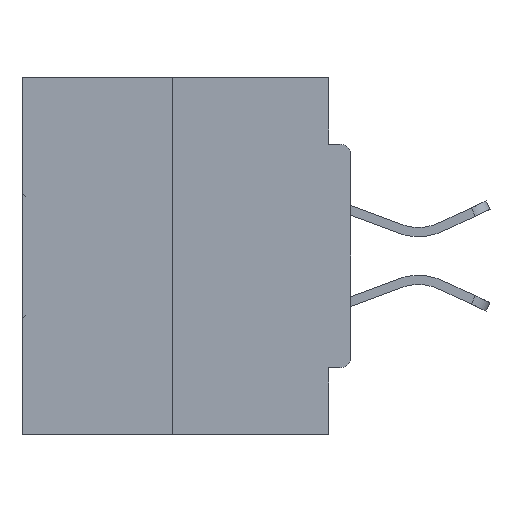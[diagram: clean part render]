
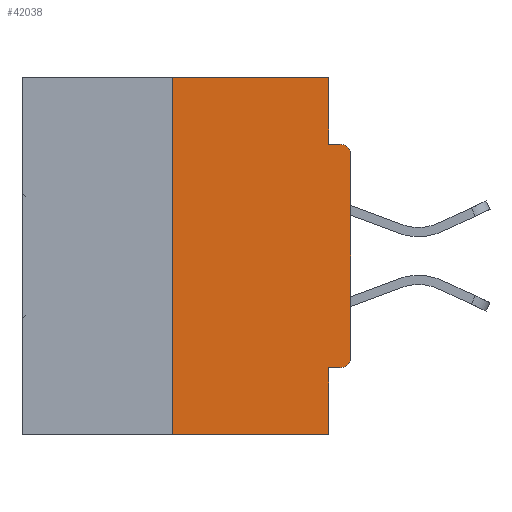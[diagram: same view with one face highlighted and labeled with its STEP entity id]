
A CAD part, left-side view. The second image highlights one B-rep face of the part: STEP entity #42038.
In plain terms, the highlighted planar face has unit normal (-1, 0, 0).
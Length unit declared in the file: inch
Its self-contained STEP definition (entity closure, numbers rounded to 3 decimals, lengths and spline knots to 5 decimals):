
#334 = DIRECTION ( 'NONE',  ( 0., 0., -1. ) ) ;
#1016 = VERTEX_POINT ( 'NONE', #9469 ) ;
#1318 = DIRECTION ( 'NONE',  ( 0., 1., 0. ) ) ;
#1459 = DIRECTION ( 'NONE',  ( 0., 0., -1. ) ) ;
#1527 = AXIS2_PLACEMENT_3D ( 'NONE', #21314, #37985, #27850 ) ;
#2402 = VERTEX_POINT ( 'NONE', #4307 ) ;
#3117 = CARTESIAN_POINT ( 'NONE',  ( 0., 0.031, 0. ) ) ;
#3133 = ORIENTED_EDGE ( 'NONE', *, *, #43009, .T. ) ;
#3311 = VECTOR ( 'NONE', #43446, 39.37008 ) ;
#3558 = ORIENTED_EDGE ( 'NONE', *, *, #34894, .F. ) ;
#3922 = PLANE ( 'NONE',  #1527 ) ;
#4307 = CARTESIAN_POINT ( 'NONE',  ( 0., 0.25, -0.5 ) ) ;
#4347 = EDGE_CURVE ( 'NONE', #12776, #28680, #35687, .T. ) ;
#4463 = ORIENTED_EDGE ( 'NONE', *, *, #4347, .T. ) ;
#5282 = EDGE_CURVE ( 'NONE', #12776, #1016, #42482, .T. ) ;
#5519 = CARTESIAN_POINT ( 'NONE',  ( 0., 0.015, -0.0935 ) ) ;
#5684 = VERTEX_POINT ( 'NONE', #11713 ) ;
#5718 = VECTOR ( 'NONE', #26559, 39.37008 ) ;
#6211 = CARTESIAN_POINT ( 'NONE',  ( 0., 0.25, 0. ) ) ;
#6405 = VECTOR ( 'NONE', #334, 39.37008 ) ;
#7506 = ORIENTED_EDGE ( 'NONE', *, *, #43290, .T. ) ;
#7690 = VERTEX_POINT ( 'NONE', #5519 ) ;
#8059 = LINE ( 'NONE', #3117, #6405 ) ;
#9285 = CARTESIAN_POINT ( 'NONE',  ( 0., 0.031, -0.5 ) ) ;
#9469 = CARTESIAN_POINT ( 'NONE',  ( 0., 0.031, -0.4065 ) ) ;
#10117 = LINE ( 'NONE', #15519, #36185 ) ;
#10723 = CARTESIAN_POINT ( 'NONE',  ( 0., 0.031, -0.5 ) ) ;
#11568 = CARTESIAN_POINT ( 'NONE',  ( 0., 0.015, -0.4065 ) ) ;
#11713 = CARTESIAN_POINT ( 'NONE',  ( 0., 0., -0.1085 ) ) ;
#12007 = CARTESIAN_POINT ( 'NONE',  ( 0., 0.031, 0. ) ) ;
#12776 = VERTEX_POINT ( 'NONE', #11568 ) ;
#13232 = EDGE_LOOP ( 'NONE', ( #34728, #21912, #25140, #3558, #31041, #4463, #7506, #3133, #35526, #29501 ) ) ;
#13595 = DIRECTION ( 'NONE',  ( -1., 0., 0. ) ) ;
#14269 = DIRECTION ( 'NONE',  ( 0., 0., -1. ) ) ;
#14966 = VERTEX_POINT ( 'NONE', #22808 ) ;
#15519 = CARTESIAN_POINT ( 'NONE',  ( 0., 0., -0.0935 ) ) ;
#16822 = CARTESIAN_POINT ( 'NONE',  ( 0., 0.46, -0.5 ) ) ;
#17137 = CIRCLE ( 'NONE', #24014, 0.015 ) ;
#18569 = DIRECTION ( 'NONE',  ( 0., -1., 0. ) ) ;
#20213 = VECTOR ( 'NONE', #43992, 39.37008 ) ;
#20291 = AXIS2_PLACEMENT_3D ( 'NONE', #22731, #13595, #14269 ) ;
#20331 = EDGE_CURVE ( 'NONE', #37708, #37813, #36535, .T. ) ;
#21314 = CARTESIAN_POINT ( 'NONE',  ( 0., 0.46, 0. ) ) ;
#21371 = DIRECTION ( 'NONE',  ( -1., 0., 0. ) ) ;
#21415 = LINE ( 'NONE', #36383, #3311 ) ;
#21912 = ORIENTED_EDGE ( 'NONE', *, *, #25961, .F. ) ;
#22731 = CARTESIAN_POINT ( 'NONE',  ( 0., 0.015, -0.3915 ) ) ;
#22808 = CARTESIAN_POINT ( 'NONE',  ( 0., 0.031, -0.0935 ) ) ;
#24014 = AXIS2_PLACEMENT_3D ( 'NONE', #24760, #21371, #1459 ) ;
#24209 = EDGE_CURVE ( 'NONE', #37813, #14966, #8059, .T. ) ;
#24553 = VECTOR ( 'NONE', #31074, 39.37008 ) ;
#24760 = CARTESIAN_POINT ( 'NONE',  ( 0., 0.015, -0.1085 ) ) ;
#25140 = ORIENTED_EDGE ( 'NONE', *, *, #35681, .T. ) ;
#25930 = VECTOR ( 'NONE', #1318, 39.37008 ) ;
#25961 = EDGE_CURVE ( 'NONE', #2402, #37708, #29664, .T. ) ;
#26559 = DIRECTION ( 'NONE',  ( 0., 0., 1. ) ) ;
#27850 = DIRECTION ( 'NONE',  ( 0., 0., -1. ) ) ;
#28288 = LINE ( 'NONE', #10723, #24553 ) ;
#28680 = VERTEX_POINT ( 'NONE', #34039 ) ;
#28784 = CARTESIAN_POINT ( 'NONE',  ( 0., 0.46, 0. ) ) ;
#28924 = EDGE_CURVE ( 'NONE', #14966, #7690, #10117, .T. ) ;
#29038 = DIRECTION ( 'NONE',  ( 0., -1., 0. ) ) ;
#29501 = ORIENTED_EDGE ( 'NONE', *, *, #24209, .F. ) ;
#29664 = LINE ( 'NONE', #6211, #5718 ) ;
#31041 = ORIENTED_EDGE ( 'NONE', *, *, #5282, .F. ) ;
#31074 = DIRECTION ( 'NONE',  ( 0., 0., -1. ) ) ;
#32377 = CARTESIAN_POINT ( 'NONE',  ( 0., 0.25, 0. ) ) ;
#32471 = LINE ( 'NONE', #16822, #20213 ) ;
#34039 = CARTESIAN_POINT ( 'NONE',  ( 0., 0., -0.3915 ) ) ;
#34728 = ORIENTED_EDGE ( 'NONE', *, *, #20331, .F. ) ;
#34894 = EDGE_CURVE ( 'NONE', #1016, #43355, #28288, .T. ) ;
#34917 = CARTESIAN_POINT ( 'NONE',  ( 0., 0., -0.4065 ) ) ;
#35526 = ORIENTED_EDGE ( 'NONE', *, *, #28924, .F. ) ;
#35681 = EDGE_CURVE ( 'NONE', #2402, #43355, #32471, .T. ) ;
#35687 = CIRCLE ( 'NONE', #20291, 0.015 ) ;
#36185 = VECTOR ( 'NONE', #29038, 39.37008 ) ;
#36383 = CARTESIAN_POINT ( 'NONE',  ( 0., 0., 0. ) ) ;
#36535 = LINE ( 'NONE', #28784, #40715 ) ;
#37708 = VERTEX_POINT ( 'NONE', #32377 ) ;
#37813 = VERTEX_POINT ( 'NONE', #12007 ) ;
#37985 = DIRECTION ( 'NONE',  ( 1., 0., 0. ) ) ;
#40715 = VECTOR ( 'NONE', #18569, 39.37008 ) ;
#42038 = ADVANCED_FACE ( 'NONE', ( #43218 ), #3922, .F. ) ;
#42482 = LINE ( 'NONE', #34917, #25930 ) ;
#43009 = EDGE_CURVE ( 'NONE', #5684, #7690, #17137, .T. ) ;
#43218 = FACE_OUTER_BOUND ( 'NONE', #13232, .T. ) ;
#43290 = EDGE_CURVE ( 'NONE', #28680, #5684, #21415, .T. ) ;
#43355 = VERTEX_POINT ( 'NONE', #9285 ) ;
#43446 = DIRECTION ( 'NONE',  ( 0., 0., 1. ) ) ;
#43992 = DIRECTION ( 'NONE',  ( 0., -1., 0. ) ) ;
